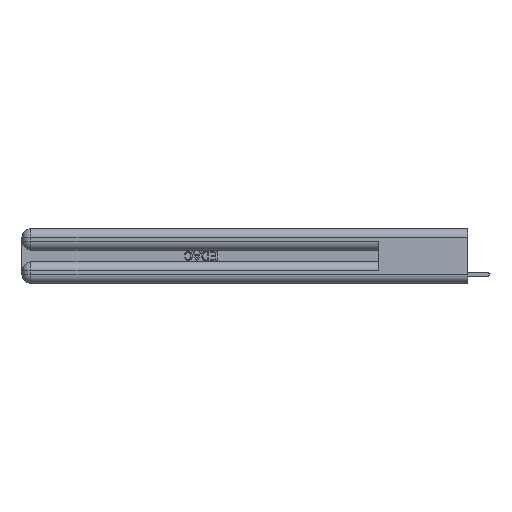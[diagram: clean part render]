
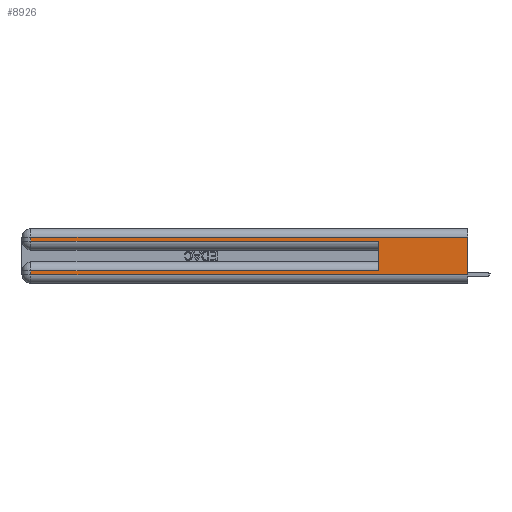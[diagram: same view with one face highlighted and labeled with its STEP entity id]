
A CAD part, left-side view. The second image highlights one B-rep face of the part: STEP entity #8926.
In plain terms, the highlighted planar face has unit normal (-1, 0, 0).
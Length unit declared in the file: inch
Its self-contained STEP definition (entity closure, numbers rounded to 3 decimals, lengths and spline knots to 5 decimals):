
#160 = CARTESIAN_POINT ( 'NONE',  ( 0., 0., 0.06 ) ) ;
#1965 = VERTEX_POINT ( 'NONE', #5758 ) ;
#2345 = EDGE_CURVE ( 'NONE', #25573, #20281, #4500, .T. ) ;
#2505 = CARTESIAN_POINT ( 'NONE',  ( 0., 2.94, 0.285 ) ) ;
#2567 = VECTOR ( 'NONE', #17484, 39.37008 ) ;
#2981 = ORIENTED_EDGE ( 'NONE', *, *, #8481, .T. ) ;
#3115 = CARTESIAN_POINT ( 'NONE',  ( 0., 0.6, 0.285 ) ) ;
#3249 = CARTESIAN_POINT ( 'NONE',  ( 0., 2.94, 0.31 ) ) ;
#3768 = VECTOR ( 'NONE', #17591, 39.37008 ) ;
#4166 = EDGE_CURVE ( 'NONE', #8075, #1965, #31030, .T. ) ;
#4500 = LINE ( 'NONE', #9740, #27013 ) ;
#5124 = DIRECTION ( 'NONE',  ( 0., 0., -1. ) ) ;
#5363 = ORIENTED_EDGE ( 'NONE', *, *, #2345, .F. ) ;
#5758 = CARTESIAN_POINT ( 'NONE',  ( 0., 2.94, 0.06 ) ) ;
#5815 = VERTEX_POINT ( 'NONE', #11431 ) ;
#5867 = CARTESIAN_POINT ( 'NONE',  ( 0., 0.6, 0.085 ) ) ;
#6323 = LINE ( 'NONE', #19663, #12373 ) ;
#6768 = CARTESIAN_POINT ( 'NONE',  ( 0., 0., 0.06 ) ) ;
#7230 = CARTESIAN_POINT ( 'NONE',  ( 0., 0., 0.37 ) ) ;
#7552 = ORIENTED_EDGE ( 'NONE', *, *, #12074, .T. ) ;
#7805 = CARTESIAN_POINT ( 'NONE',  ( 0., 0., 0.285 ) ) ;
#8007 = CARTESIAN_POINT ( 'NONE',  ( 0., 0., 0.37 ) ) ;
#8075 = VERTEX_POINT ( 'NONE', #18020 ) ;
#8127 = EDGE_CURVE ( 'NONE', #25573, #8075, #21679, .T. ) ;
#8424 = EDGE_LOOP ( 'NONE', ( #10339, #9074, #2981, #10443, #5363, #29904, #19722, #7552 ) ) ;
#8481 = EDGE_CURVE ( 'NONE', #22080, #28563, #31213, .T. ) ;
#8926 = ADVANCED_FACE ( 'NONE', ( #10640 ), #26245, .F. ) ;
#9074 = ORIENTED_EDGE ( 'NONE', *, *, #22987, .T. ) ;
#9570 = VECTOR ( 'NONE', #5124, 39.37008 ) ;
#9740 = CARTESIAN_POINT ( 'NONE',  ( 0., 0.6, 0.145 ) ) ;
#10339 = ORIENTED_EDGE ( 'NONE', *, *, #10872, .F. ) ;
#10443 = ORIENTED_EDGE ( 'NONE', *, *, #12311, .T. ) ;
#10640 = FACE_OUTER_BOUND ( 'NONE', #8424, .T. ) ;
#10872 = EDGE_CURVE ( 'NONE', #5815, #30016, #31220, .T. ) ;
#11431 = CARTESIAN_POINT ( 'NONE',  ( 0., 0., 0.31 ) ) ;
#12074 = EDGE_CURVE ( 'NONE', #1965, #30016, #17317, .T. ) ;
#12311 = EDGE_CURVE ( 'NONE', #28563, #20281, #31795, .T. ) ;
#12373 = VECTOR ( 'NONE', #27679, 39.37008 ) ;
#16283 = VECTOR ( 'NONE', #17954, 39.37008 ) ;
#16611 = VECTOR ( 'NONE', #18877, 39.37008 ) ;
#17317 = LINE ( 'NONE', #6768, #2567 ) ;
#17484 = DIRECTION ( 'NONE',  ( 0., -1., 0. ) ) ;
#17591 = DIRECTION ( 'NONE',  ( 0., 0., -1. ) ) ;
#17954 = DIRECTION ( 'NONE',  ( 0., 0., -1. ) ) ;
#18020 = CARTESIAN_POINT ( 'NONE',  ( 0., 2.94, 0.085 ) ) ;
#18877 = DIRECTION ( 'NONE',  ( 0., -1., 0. ) ) ;
#19663 = CARTESIAN_POINT ( 'NONE',  ( 0., 0., 0.31 ) ) ;
#19722 = ORIENTED_EDGE ( 'NONE', *, *, #4166, .T. ) ;
#20217 = CARTESIAN_POINT ( 'NONE',  ( 0., 0., 0.085 ) ) ;
#20281 = VERTEX_POINT ( 'NONE', #3115 ) ;
#21172 = DIRECTION ( 'NONE',  ( 0., 0., -1. ) ) ;
#21679 = LINE ( 'NONE', #20217, #32920 ) ;
#22080 = VERTEX_POINT ( 'NONE', #3249 ) ;
#22987 = EDGE_CURVE ( 'NONE', #5815, #22080, #6323, .T. ) ;
#23607 = DIRECTION ( 'NONE',  ( 1., 0., 0. ) ) ;
#25573 = VERTEX_POINT ( 'NONE', #5867 ) ;
#26245 = PLANE ( 'NONE',  #28128 ) ;
#27013 = VECTOR ( 'NONE', #28670, 39.37008 ) ;
#27093 = DIRECTION ( 'NONE',  ( 0., 1., 0. ) ) ;
#27679 = DIRECTION ( 'NONE',  ( 0., 1., 0. ) ) ;
#28128 = AXIS2_PLACEMENT_3D ( 'NONE', #8007, #23607, #21172 ) ;
#28563 = VERTEX_POINT ( 'NONE', #2505 ) ;
#28670 = DIRECTION ( 'NONE',  ( 0., 0., 1. ) ) ;
#29126 = CARTESIAN_POINT ( 'NONE',  ( 0., 2.94, 0.37 ) ) ;
#29904 = ORIENTED_EDGE ( 'NONE', *, *, #8127, .T. ) ;
#30016 = VERTEX_POINT ( 'NONE', #160 ) ;
#31030 = LINE ( 'NONE', #34006, #3768 ) ;
#31213 = LINE ( 'NONE', #29126, #9570 ) ;
#31220 = LINE ( 'NONE', #7230, #16283 ) ;
#31795 = LINE ( 'NONE', #7805, #16611 ) ;
#32920 = VECTOR ( 'NONE', #27093, 39.37008 ) ;
#34006 = CARTESIAN_POINT ( 'NONE',  ( 0., 2.94, 0.37 ) ) ;
